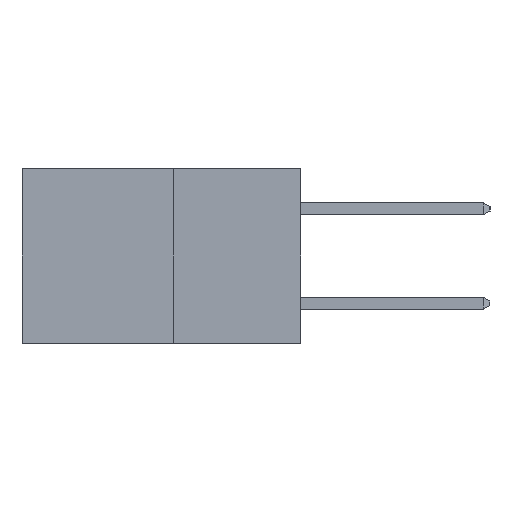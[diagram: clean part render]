
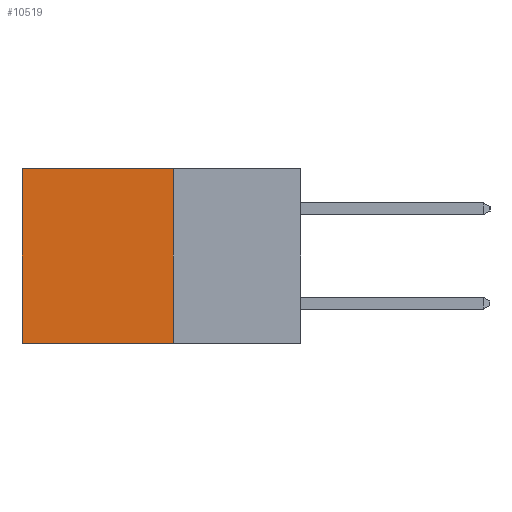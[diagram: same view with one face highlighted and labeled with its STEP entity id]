
A CAD part, left-side view. The second image highlights one B-rep face of the part: STEP entity #10519.
In plain terms, the highlighted planar face has unit normal (-1, 0, 0).
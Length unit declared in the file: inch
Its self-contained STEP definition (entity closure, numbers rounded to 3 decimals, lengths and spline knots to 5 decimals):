
#443 = DIRECTION ( 'NONE',  ( 1., 0., 0. ) ) ;
#1102 = EDGE_CURVE ( 'NONE', #5709, #3636, #10490, .T. ) ;
#1892 = VECTOR ( 'NONE', #3437, 39.37008 ) ;
#2048 = CARTESIAN_POINT ( 'NONE',  ( 0.277, 0.59, -0.37 ) ) ;
#3021 = DIRECTION ( 'NONE',  ( 0., 0., -1. ) ) ;
#3437 = DIRECTION ( 'NONE',  ( 0., 0., -1. ) ) ;
#3636 = VERTEX_POINT ( 'NONE', #3663 ) ;
#3663 = CARTESIAN_POINT ( 'NONE',  ( 0.277, 0.59, 0. ) ) ;
#4605 = EDGE_CURVE ( 'NONE', #3636, #10590, #12394, .T. ) ;
#5288 = VECTOR ( 'NONE', #3021, 39.37008 ) ;
#5422 = FACE_OUTER_BOUND ( 'NONE', #12710, .T. ) ;
#5709 = VERTEX_POINT ( 'NONE', #13693 ) ;
#5813 = ORIENTED_EDGE ( 'NONE', *, *, #1102, .T. ) ;
#5906 = CARTESIAN_POINT ( 'NONE',  ( 0.277, 0.27, 0. ) ) ;
#5960 = ORIENTED_EDGE ( 'NONE', *, *, #4605, .T. ) ;
#6141 = CARTESIAN_POINT ( 'NONE',  ( 0.277, 0.27, -0.37 ) ) ;
#6343 = ORIENTED_EDGE ( 'NONE', *, *, #15099, .F. ) ;
#6550 = DIRECTION ( 'NONE',  ( 0., 1., 0. ) ) ;
#6709 = LINE ( 'NONE', #6141, #10086 ) ;
#8042 = EDGE_CURVE ( 'NONE', #16203, #10590, #6709, .T. ) ;
#8740 = CARTESIAN_POINT ( 'NONE',  ( 0.277, 0.59, -0.37 ) ) ;
#9885 = DIRECTION ( 'NONE',  ( 0., 0., -1. ) ) ;
#9905 = ORIENTED_EDGE ( 'NONE', *, *, #8042, .F. ) ;
#10086 = VECTOR ( 'NONE', #13712, 39.37008 ) ;
#10490 = LINE ( 'NONE', #5906, #13839 ) ;
#10519 = ADVANCED_FACE ( 'NONE', ( #5422 ), #16010, .F. ) ;
#10590 = VERTEX_POINT ( 'NONE', #8740 ) ;
#12394 = LINE ( 'NONE', #2048, #1892 ) ;
#12581 = CARTESIAN_POINT ( 'NONE',  ( 0.277, 0.27, -0.37 ) ) ;
#12710 = EDGE_LOOP ( 'NONE', ( #5960, #9905, #6343, #5813 ) ) ;
#13693 = CARTESIAN_POINT ( 'NONE',  ( 0.277, 0.27, 0. ) ) ;
#13712 = DIRECTION ( 'NONE',  ( 0., 1., 0. ) ) ;
#13839 = VECTOR ( 'NONE', #6550, 39.37008 ) ;
#14610 = AXIS2_PLACEMENT_3D ( 'NONE', #16066, #443, #9885 ) ;
#15099 = EDGE_CURVE ( 'NONE', #5709, #16203, #15372, .T. ) ;
#15372 = LINE ( 'NONE', #15852, #5288 ) ;
#15852 = CARTESIAN_POINT ( 'NONE',  ( 0.277, 0.27, -0.37 ) ) ;
#16010 = PLANE ( 'NONE',  #14610 ) ;
#16066 = CARTESIAN_POINT ( 'NONE',  ( 0.277, 0.27, -0.37 ) ) ;
#16203 = VERTEX_POINT ( 'NONE', #12581 ) ;
